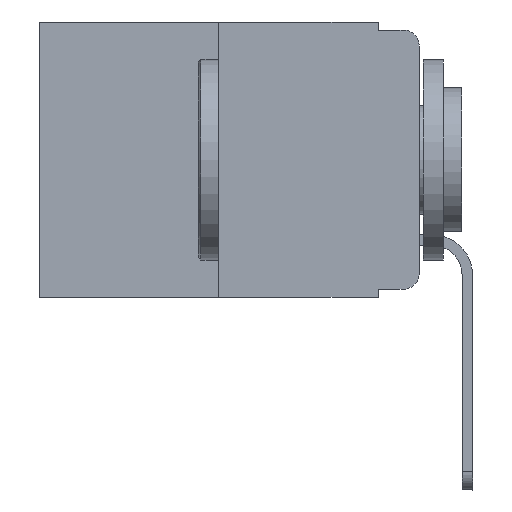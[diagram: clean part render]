
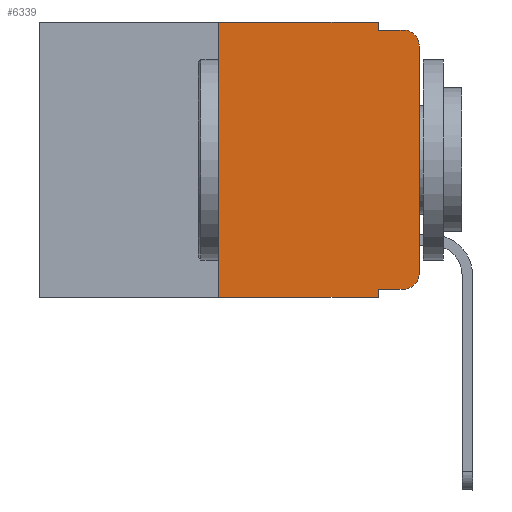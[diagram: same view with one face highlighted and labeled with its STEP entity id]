
A CAD part, left-side view. The second image highlights one B-rep face of the part: STEP entity #6339.
In plain terms, the highlighted planar face has unit normal (-1, 0, 0).
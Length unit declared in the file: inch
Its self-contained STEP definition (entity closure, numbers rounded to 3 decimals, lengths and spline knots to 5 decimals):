
#168 = CARTESIAN_POINT ( 'NONE',  ( 0., 0.051, 0. ) ) ;
#380 = DIRECTION ( 'NONE',  ( 0., 0., -1. ) ) ;
#480 = CARTESIAN_POINT ( 'NONE',  ( 0., 0.02, -0.333 ) ) ;
#570 = DIRECTION ( 'NONE',  ( 0., 0., 1. ) ) ;
#869 = AXIS2_PLACEMENT_3D ( 'NONE', #2348, #9188, #380 ) ;
#987 = ORIENTED_EDGE ( 'NONE', *, *, #5165, .T. ) ;
#1008 = EDGE_LOOP ( 'NONE', ( #10774, #987, #11817, #9356, #1954, #7706, #12909, #4047, #8154, #10618 ) ) ;
#1019 = EDGE_CURVE ( 'NONE', #11182, #12493, #10514, .T. ) ;
#1511 = CARTESIAN_POINT ( 'NONE',  ( 0., 0., -0.03 ) ) ;
#1607 = VECTOR ( 'NONE', #8579, 39.37008 ) ;
#1654 = VERTEX_POINT ( 'NONE', #5228 ) ;
#1954 = ORIENTED_EDGE ( 'NONE', *, *, #7868, .F. ) ;
#2296 = VECTOR ( 'NONE', #8298, 39.37008 ) ;
#2335 = VECTOR ( 'NONE', #4152, 39.37008 ) ;
#2348 = CARTESIAN_POINT ( 'NONE',  ( 0., 0.02, -0.313 ) ) ;
#2390 = DIRECTION ( 'NONE',  ( 0., -1., 0. ) ) ;
#2728 = DIRECTION ( 'NONE',  ( -1., 0., 0. ) ) ;
#2753 = AXIS2_PLACEMENT_3D ( 'NONE', #11718, #2728, #6758 ) ;
#3231 = DIRECTION ( 'NONE',  ( 0., -1., 0. ) ) ;
#3376 = DIRECTION ( 'NONE',  ( 0., 0., -1. ) ) ;
#3996 = CARTESIAN_POINT ( 'NONE',  ( 0., 0.051, -0.01 ) ) ;
#4035 = LINE ( 'NONE', #11229, #9446 ) ;
#4047 = ORIENTED_EDGE ( 'NONE', *, *, #10931, .F. ) ;
#4074 = CARTESIAN_POINT ( 'NONE',  ( 0., 0.25, -0.343 ) ) ;
#4152 = DIRECTION ( 'NONE',  ( 0., 0., 1. ) ) ;
#4163 = CARTESIAN_POINT ( 'NONE',  ( 0., 0.051, -0.333 ) ) ;
#4310 = VECTOR ( 'NONE', #12122, 39.37008 ) ;
#4422 = LINE ( 'NONE', #4163, #2296 ) ;
#4627 = DIRECTION ( 'NONE',  ( 1., 0., 0. ) ) ;
#4779 = CARTESIAN_POINT ( 'NONE',  ( 0., 0.051, -0.343 ) ) ;
#5165 = EDGE_CURVE ( 'NONE', #9454, #9736, #10927, .T. ) ;
#5168 = VERTEX_POINT ( 'NONE', #4779 ) ;
#5228 = CARTESIAN_POINT ( 'NONE',  ( 0., 0.051, -0.333 ) ) ;
#5503 = CARTESIAN_POINT ( 'NONE',  ( 0., 0.051, 0. ) ) ;
#5556 = CARTESIAN_POINT ( 'NONE',  ( 0., 0.473, 0. ) ) ;
#5584 = CARTESIAN_POINT ( 'NONE',  ( 0., 0.25, 0. ) ) ;
#5925 = EDGE_CURVE ( 'NONE', #11356, #11187, #6683, .T. ) ;
#6339 = ADVANCED_FACE ( 'NONE', ( #10517 ), #8508, .F. ) ;
#6683 = LINE ( 'NONE', #5503, #1607 ) ;
#6758 = DIRECTION ( 'NONE',  ( 0., 0., -1. ) ) ;
#7408 = CARTESIAN_POINT ( 'NONE',  ( 0., 0.473, -0.343 ) ) ;
#7671 = LINE ( 'NONE', #5584, #12228 ) ;
#7701 = CARTESIAN_POINT ( 'NONE',  ( 0., 0.25, 0. ) ) ;
#7706 = ORIENTED_EDGE ( 'NONE', *, *, #10189, .F. ) ;
#7868 = EDGE_CURVE ( 'NONE', #11113, #11356, #4035, .T. ) ;
#8049 = VECTOR ( 'NONE', #2390, 39.37008 ) ;
#8154 = ORIENTED_EDGE ( 'NONE', *, *, #12669, .T. ) ;
#8298 = DIRECTION ( 'NONE',  ( 0., -1., 0. ) ) ;
#8312 = EDGE_CURVE ( 'NONE', #12493, #9454, #11084, .T. ) ;
#8508 = PLANE ( 'NONE',  #8870 ) ;
#8579 = DIRECTION ( 'NONE',  ( 0., 0., -1. ) ) ;
#8863 = VERTEX_POINT ( 'NONE', #4074 ) ;
#8870 = AXIS2_PLACEMENT_3D ( 'NONE', #5556, #4627, #12431 ) ;
#9188 = DIRECTION ( 'NONE',  ( -1., 0., 0. ) ) ;
#9356 = ORIENTED_EDGE ( 'NONE', *, *, #5925, .F. ) ;
#9446 = VECTOR ( 'NONE', #3231, 39.37008 ) ;
#9454 = VERTEX_POINT ( 'NONE', #1511 ) ;
#9660 = CARTESIAN_POINT ( 'NONE',  ( 0., 0.051, -0.01 ) ) ;
#9736 = VERTEX_POINT ( 'NONE', #10875 ) ;
#10174 = CARTESIAN_POINT ( 'NONE',  ( 0., 0., 0. ) ) ;
#10189 = EDGE_CURVE ( 'NONE', #8863, #11113, #7671, .T. ) ;
#10514 = CIRCLE ( 'NONE', #869, 0.02 ) ;
#10517 = FACE_OUTER_BOUND ( 'NONE', #1008, .T. ) ;
#10550 = CARTESIAN_POINT ( 'NONE',  ( 0., 0.051, 0. ) ) ;
#10618 = ORIENTED_EDGE ( 'NONE', *, *, #1019, .T. ) ;
#10774 = ORIENTED_EDGE ( 'NONE', *, *, #8312, .T. ) ;
#10875 = CARTESIAN_POINT ( 'NONE',  ( 0., 0.02, -0.01 ) ) ;
#10927 = CIRCLE ( 'NONE', #2753, 0.02 ) ;
#10931 = EDGE_CURVE ( 'NONE', #1654, #5168, #11183, .T. ) ;
#11084 = LINE ( 'NONE', #10174, #2335 ) ;
#11113 = VERTEX_POINT ( 'NONE', #7701 ) ;
#11180 = VECTOR ( 'NONE', #3376, 39.37008 ) ;
#11182 = VERTEX_POINT ( 'NONE', #480 ) ;
#11183 = LINE ( 'NONE', #168, #11180 ) ;
#11187 = VERTEX_POINT ( 'NONE', #9660 ) ;
#11229 = CARTESIAN_POINT ( 'NONE',  ( 0., 0.473, 0. ) ) ;
#11356 = VERTEX_POINT ( 'NONE', #10550 ) ;
#11569 = CARTESIAN_POINT ( 'NONE',  ( 0., 0., -0.313 ) ) ;
#11718 = CARTESIAN_POINT ( 'NONE',  ( 0., 0.02, -0.03 ) ) ;
#11746 = EDGE_CURVE ( 'NONE', #11187, #9736, #12964, .T. ) ;
#11817 = ORIENTED_EDGE ( 'NONE', *, *, #11746, .F. ) ;
#12122 = DIRECTION ( 'NONE',  ( 0., -1., 0. ) ) ;
#12228 = VECTOR ( 'NONE', #570, 39.37008 ) ;
#12350 = EDGE_CURVE ( 'NONE', #8863, #5168, #12367, .T. ) ;
#12367 = LINE ( 'NONE', #7408, #8049 ) ;
#12431 = DIRECTION ( 'NONE',  ( 0., 0., -1. ) ) ;
#12493 = VERTEX_POINT ( 'NONE', #11569 ) ;
#12669 = EDGE_CURVE ( 'NONE', #1654, #11182, #4422, .T. ) ;
#12909 = ORIENTED_EDGE ( 'NONE', *, *, #12350, .T. ) ;
#12964 = LINE ( 'NONE', #3996, #4310 ) ;
